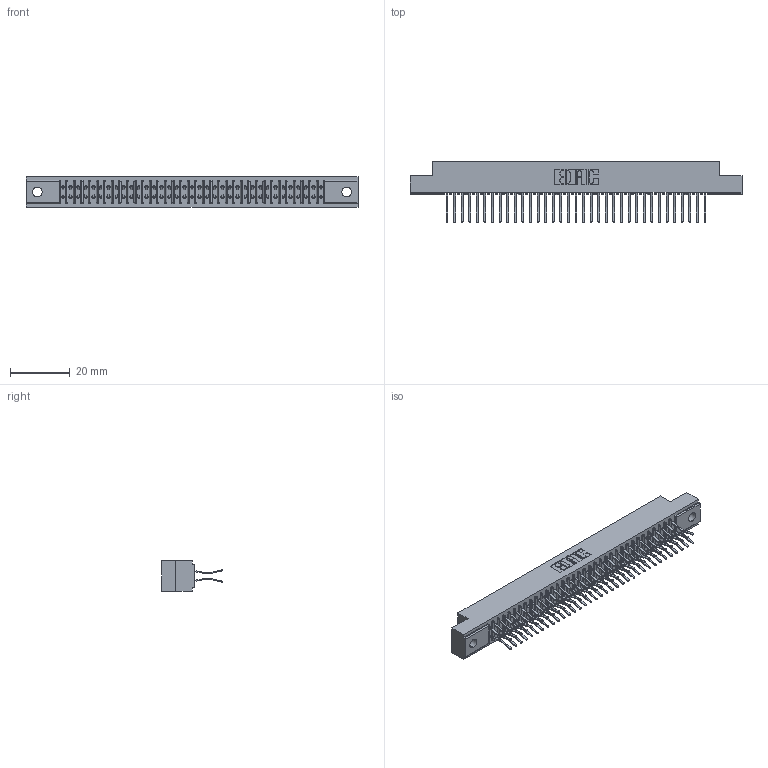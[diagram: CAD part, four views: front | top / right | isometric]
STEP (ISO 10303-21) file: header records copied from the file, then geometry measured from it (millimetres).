
FILE_DESCRIPTION (( 'STEP AP203' ), '1' );
FILE_NAME ('341-070-560-202.STEP', '2018-08-07T19:42:33', ( '' ), ( '' ), 'SwSTEP 2.0', 'SolidWorks 2016', '' );
FILE_SCHEMA (( 'CONFIG_CONTROL_DESIGN' ));
Length unit declared in the file: inch
Products named in the file (3): 341-070-560-202; 341 Part_.128 (3.25) Dia Mounting Holes; 341-292-001_341-292-160
Assembly tree (71 placements, depth 2):
  341-070-560-202
    341 Part_.128 (3.25) Dia Mounting Holes
    341-292-001_341-292-160  x70
Bounding box: 111.12 x 20.37 x 10.16 mm (x, y, z)
Volume: 8229.2 mm3; surface area: 14654.2 mm2
Topology: 71 solids, 71 shells, 5016 faces, 14561 edges, 9446 vertices
Faces by surface type: plane 2868, cylinder 2008, sphere 72, torus 68
Entity records: 43432 total; most frequent: CARTESIAN_POINT 7221, ORIENTED_EDGE 7174, DIRECTION 7017, EDGE_CURVE 3587, LINE 2885, VECTOR 2885, VERTEX_POINT 2270, AXIS2_PLACEMENT_3D 2066
